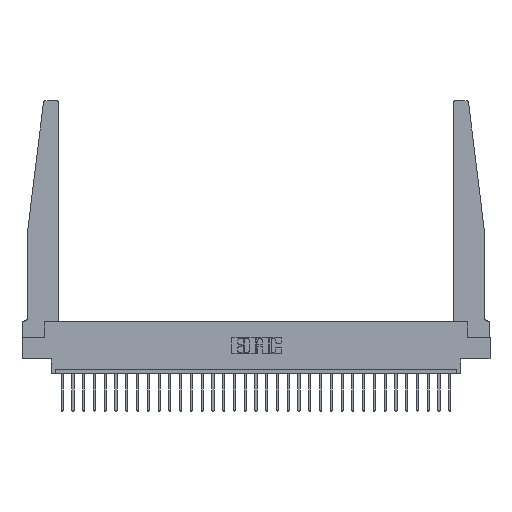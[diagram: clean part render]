
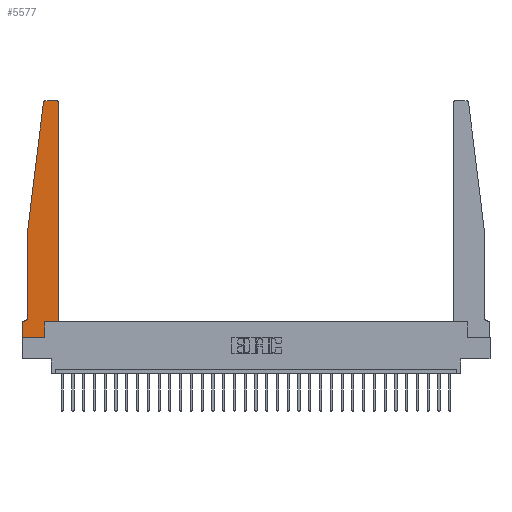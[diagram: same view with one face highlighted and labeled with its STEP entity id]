
A CAD part, top view. The second image highlights one B-rep face of the part: STEP entity #5577.
In plain terms, the highlighted planar face has unit normal (0, 0, 1).
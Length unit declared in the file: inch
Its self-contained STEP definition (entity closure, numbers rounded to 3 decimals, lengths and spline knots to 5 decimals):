
#68 = ORIENTED_EDGE ( 'NONE', *, *, #15807, .T. ) ;
#70 = ORIENTED_EDGE ( 'NONE', *, *, #6232, .T. ) ;
#178 = AXIS2_PLACEMENT_3D ( 'NONE', #16071, #4649, #9464 ) ;
#188 = CARTESIAN_POINT ( 'NONE',  ( 0.015, 0.2375, 0.37 ) ) ;
#386 = DIRECTION ( 'NONE',  ( 0., 1., 0. ) ) ;
#390 = DIRECTION ( 'NONE',  ( 0., 0., -1. ) ) ;
#725 = ORIENTED_EDGE ( 'NONE', *, *, #18395, .T. ) ;
#1026 = CARTESIAN_POINT ( 'NONE',  ( 0.2605, 0.18, 0.37 ) ) ;
#1042 = VERTEX_POINT ( 'NONE', #8292 ) ;
#1499 = CARTESIAN_POINT ( 'NONE',  ( 0., 0.1875, 0.37 ) ) ;
#1876 = DIRECTION ( 'NONE',  ( 0., 1., 0. ) ) ;
#2087 = DIRECTION ( 'NONE',  ( 1., 0., 0. ) ) ;
#2263 = DIRECTION ( 'NONE',  ( 0., 0., 1. ) ) ;
#2409 = LINE ( 'NONE', #11818, #3811 ) ;
#2502 = DIRECTION ( 'NONE',  ( -1., 0., 0. ) ) ;
#2748 = EDGE_LOOP ( 'NONE', ( #21038, #725, #26629, #24886, #15659, #70, #14249, #19624, #68, #13241, #24088, #27230 ) ) ;
#2751 = CARTESIAN_POINT ( 'NONE',  ( 0.27653, 2.72, 0.37 ) ) ;
#2787 = LINE ( 'NONE', #28282, #4510 ) ;
#3000 = VECTOR ( 'NONE', #16337, 39.37008 ) ;
#3695 = VECTOR ( 'NONE', #25018, 39.37008 ) ;
#3811 = VECTOR ( 'NONE', #14055, 39.37008 ) ;
#4058 = DIRECTION ( 'NONE',  ( -0.122, -0.992, 0. ) ) ;
#4452 = CARTESIAN_POINT ( 'NONE',  ( 0.425, 0.18, 0.37 ) ) ;
#4510 = VECTOR ( 'NONE', #1876, 39.37008 ) ;
#4649 = DIRECTION ( 'NONE',  ( 0., 0., 1. ) ) ;
#4935 = VERTEX_POINT ( 'NONE', #15039 ) ;
#5577 = ADVANCED_FACE ( 'NONE', ( #21184 ), #15973, .T. ) ;
#5602 = LINE ( 'NONE', #26006, #27311 ) ;
#6227 = EDGE_CURVE ( 'NONE', #1042, #16471, #12851, .T. ) ;
#6232 = EDGE_CURVE ( 'NONE', #6253, #17753, #23535, .T. ) ;
#6253 = VERTEX_POINT ( 'NONE', #6286 ) ;
#6286 = CARTESIAN_POINT ( 'NONE',  ( 0.015, 0.1875, 0.37 ) ) ;
#6919 = LINE ( 'NONE', #23111, #15589 ) ;
#7034 = CARTESIAN_POINT ( 'NONE',  ( 0.2605, 0., 0.37 ) ) ;
#7206 = DIRECTION ( 'NONE',  ( 0., 0., 1. ) ) ;
#7323 = CARTESIAN_POINT ( 'NONE',  ( 0.065, 1.25, 0.37 ) ) ;
#7496 = CARTESIAN_POINT ( 'NONE',  ( 0., 0., 0.37 ) ) ;
#7881 = EDGE_CURVE ( 'NONE', #9641, #13498, #2409, .T. ) ;
#8238 = CIRCLE ( 'NONE', #21747, 0.05 ) ;
#8292 = CARTESIAN_POINT ( 'NONE',  ( 0.24675, 2.72367, 0.37 ) ) ;
#8683 = LINE ( 'NONE', #27075, #19069 ) ;
#9464 = DIRECTION ( 'NONE',  ( 1., 0., 0. ) ) ;
#9641 = VERTEX_POINT ( 'NONE', #18053 ) ;
#9733 = DIRECTION ( 'NONE',  ( 0., -1., 0. ) ) ;
#9799 = VERTEX_POINT ( 'NONE', #14073 ) ;
#9809 = DIRECTION ( 'NONE',  ( 1., 0., 0. ) ) ;
#9820 = AXIS2_PLACEMENT_3D ( 'NONE', #2751, #7206, #9809 ) ;
#10635 = CARTESIAN_POINT ( 'NONE',  ( 0.065, 0.1875, 0.37 ) ) ;
#11818 = CARTESIAN_POINT ( 'NONE',  ( 0.25, 2.75, 0.37 ) ) ;
#12513 = VECTOR ( 'NONE', #28241, 39.37008 ) ;
#12827 = DIRECTION ( 'NONE',  ( 1., 0., 0. ) ) ;
#12851 = LINE ( 'NONE', #12863, #18035 ) ;
#12863 = CARTESIAN_POINT ( 'NONE',  ( 0.065, 1.25, 0.37 ) ) ;
#13151 = VERTEX_POINT ( 'NONE', #7034 ) ;
#13189 = CIRCLE ( 'NONE', #9820, 0.03 ) ;
#13241 = ORIENTED_EDGE ( 'NONE', *, *, #21258, .T. ) ;
#13498 = VERTEX_POINT ( 'NONE', #22623 ) ;
#13720 = EDGE_CURVE ( 'NONE', #4935, #13151, #21363, .T. ) ;
#14055 = DIRECTION ( 'NONE',  ( -1., 0., 0. ) ) ;
#14073 = CARTESIAN_POINT ( 'NONE',  ( 0.065, 0.2375, 0.37 ) ) ;
#14249 = ORIENTED_EDGE ( 'NONE', *, *, #22411, .T. ) ;
#15004 = VERTEX_POINT ( 'NONE', #1026 ) ;
#15039 = CARTESIAN_POINT ( 'NONE',  ( 0., 0., 0.37 ) ) ;
#15589 = VECTOR ( 'NONE', #9733, 39.37008 ) ;
#15659 = ORIENTED_EDGE ( 'NONE', *, *, #23405, .T. ) ;
#15807 = EDGE_CURVE ( 'NONE', #13151, #15004, #2787, .T. ) ;
#15973 = PLANE ( 'NONE',  #178 ) ;
#16071 = CARTESIAN_POINT ( 'NONE',  ( 0., 0.1875, 0.37 ) ) ;
#16337 = DIRECTION ( 'NONE',  ( 0., -1., 0. ) ) ;
#16471 = VERTEX_POINT ( 'NONE', #20295 ) ;
#17753 = VERTEX_POINT ( 'NONE', #1499 ) ;
#18035 = VECTOR ( 'NONE', #4058, 39.37008 ) ;
#18053 = CARTESIAN_POINT ( 'NONE',  ( 0.395, 2.75, 0.37 ) ) ;
#18395 = EDGE_CURVE ( 'NONE', #13498, #1042, #13189, .T. ) ;
#19069 = VECTOR ( 'NONE', #386, 39.37008 ) ;
#19624 = ORIENTED_EDGE ( 'NONE', *, *, #13720, .T. ) ;
#19863 = CARTESIAN_POINT ( 'NONE',  ( 0.395, 2.72, 0.37 ) ) ;
#20061 = VERTEX_POINT ( 'NONE', #23474 ) ;
#20295 = CARTESIAN_POINT ( 'NONE',  ( 0.065, 1.25, 0.37 ) ) ;
#21038 = ORIENTED_EDGE ( 'NONE', *, *, #7881, .T. ) ;
#21184 = FACE_OUTER_BOUND ( 'NONE', #2748, .T. ) ;
#21258 = EDGE_CURVE ( 'NONE', #15004, #26921, #5602, .T. ) ;
#21363 = LINE ( 'NONE', #7496, #3695 ) ;
#21747 = AXIS2_PLACEMENT_3D ( 'NONE', #188, #390, #2502 ) ;
#22411 = EDGE_CURVE ( 'NONE', #17753, #4935, #6919, .T. ) ;
#22623 = CARTESIAN_POINT ( 'NONE',  ( 0.27653, 2.75, 0.37 ) ) ;
#23111 = CARTESIAN_POINT ( 'NONE',  ( 0., 0., 0.37 ) ) ;
#23405 = EDGE_CURVE ( 'NONE', #9799, #6253, #8238, .T. ) ;
#23474 = CARTESIAN_POINT ( 'NONE',  ( 0.425, 2.72, 0.37 ) ) ;
#23535 = LINE ( 'NONE', #10635, #12513 ) ;
#23708 = CIRCLE ( 'NONE', #26490, 0.03 ) ;
#23993 = EDGE_CURVE ( 'NONE', #16471, #9799, #27137, .T. ) ;
#24088 = ORIENTED_EDGE ( 'NONE', *, *, #27098, .T. ) ;
#24395 = EDGE_CURVE ( 'NONE', #20061, #9641, #23708, .T. ) ;
#24886 = ORIENTED_EDGE ( 'NONE', *, *, #23993, .T. ) ;
#25018 = DIRECTION ( 'NONE',  ( 1., 0., 0. ) ) ;
#26006 = CARTESIAN_POINT ( 'NONE',  ( 0.425, 0.18, 0.37 ) ) ;
#26490 = AXIS2_PLACEMENT_3D ( 'NONE', #19863, #2263, #2087 ) ;
#26629 = ORIENTED_EDGE ( 'NONE', *, *, #6227, .T. ) ;
#26921 = VERTEX_POINT ( 'NONE', #4452 ) ;
#27075 = CARTESIAN_POINT ( 'NONE',  ( 0.425, 0.18, 0.37 ) ) ;
#27098 = EDGE_CURVE ( 'NONE', #26921, #20061, #8683, .T. ) ;
#27137 = LINE ( 'NONE', #7323, #3000 ) ;
#27230 = ORIENTED_EDGE ( 'NONE', *, *, #24395, .T. ) ;
#27311 = VECTOR ( 'NONE', #12827, 39.37008 ) ;
#28241 = DIRECTION ( 'NONE',  ( -1., 0., 0. ) ) ;
#28282 = CARTESIAN_POINT ( 'NONE',  ( 0.2605, 0.18, 0.37 ) ) ;
